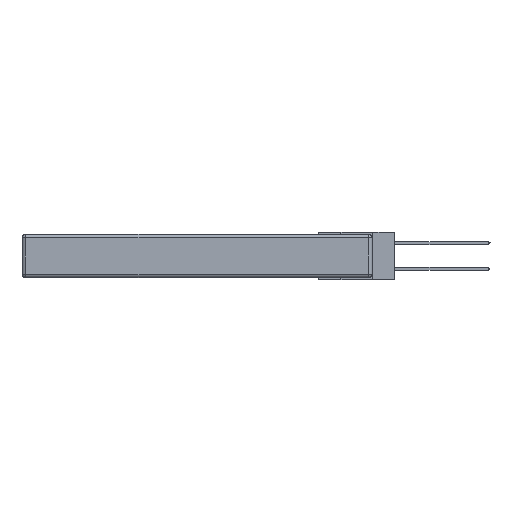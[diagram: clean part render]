
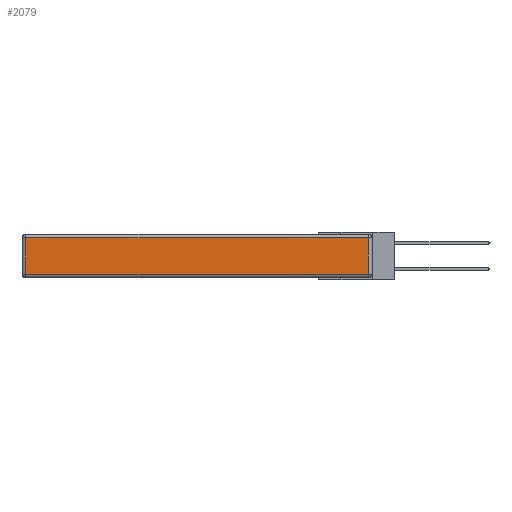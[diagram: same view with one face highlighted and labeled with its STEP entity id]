
A CAD part, left-side view. The second image highlights one B-rep face of the part: STEP entity #2079.
In plain terms, the highlighted planar face has unit normal (-1, 0, 0).
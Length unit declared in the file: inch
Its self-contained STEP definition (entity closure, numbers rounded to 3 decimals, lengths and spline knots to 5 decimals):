
#499 = DIRECTION ( 'NONE',  ( 0., 0., 1. ) ) ;
#761 = CARTESIAN_POINT ( 'NONE',  ( 0., 2.72, -0.313 ) ) ;
#2079 = ADVANCED_FACE ( 'NONE', ( #4059 ), #2693, .T. ) ;
#2693 = PLANE ( 'NONE',  #6199 ) ;
#4059 = FACE_OUTER_BOUND ( 'NONE', #22224, .T. ) ;
#5802 = DIRECTION ( 'NONE',  ( 0., 0., 1. ) ) ;
#6199 = AXIS2_PLACEMENT_3D ( 'NONE', #31024, #28366, #499 ) ;
#7087 = DIRECTION ( 'NONE',  ( 0., -1., 0. ) ) ;
#8063 = ORIENTED_EDGE ( 'NONE', *, *, #14645, .T. ) ;
#8081 = VECTOR ( 'NONE', #24309, 39.37008 ) ;
#8719 = CARTESIAN_POINT ( 'NONE',  ( 0., 0.03, -0.343 ) ) ;
#12425 = EDGE_CURVE ( 'NONE', #27812, #23654, #19739, .T. ) ;
#12857 = LINE ( 'NONE', #17059, #8081 ) ;
#12929 = LINE ( 'NONE', #8719, #15340 ) ;
#13012 = EDGE_CURVE ( 'NONE', #16909, #23980, #12929, .T. ) ;
#13393 = VECTOR ( 'NONE', #31324, 39.37008 ) ;
#14645 = EDGE_CURVE ( 'NONE', #23980, #27812, #12857, .T. ) ;
#15340 = VECTOR ( 'NONE', #5802, 39.37008 ) ;
#16909 = VERTEX_POINT ( 'NONE', #29527 ) ;
#17059 = CARTESIAN_POINT ( 'NONE',  ( 0., 2.75, -0.03 ) ) ;
#18660 = CARTESIAN_POINT ( 'NONE',  ( 0., 2.72, -0.343 ) ) ;
#19739 = LINE ( 'NONE', #18660, #13393 ) ;
#22224 = EDGE_LOOP ( 'NONE', ( #26022, #25964, #8063, #29429 ) ) ;
#22317 = CARTESIAN_POINT ( 'NONE',  ( 0., 0., -0.313 ) ) ;
#22921 = CARTESIAN_POINT ( 'NONE',  ( 0., 2.72, -0.03 ) ) ;
#23654 = VERTEX_POINT ( 'NONE', #761 ) ;
#23980 = VERTEX_POINT ( 'NONE', #29792 ) ;
#24309 = DIRECTION ( 'NONE',  ( 0., 1., 0. ) ) ;
#24898 = VECTOR ( 'NONE', #7087, 39.37008 ) ;
#25316 = LINE ( 'NONE', #22317, #24898 ) ;
#25964 = ORIENTED_EDGE ( 'NONE', *, *, #13012, .T. ) ;
#26022 = ORIENTED_EDGE ( 'NONE', *, *, #26476, .T. ) ;
#26476 = EDGE_CURVE ( 'NONE', #23654, #16909, #25316, .T. ) ;
#27812 = VERTEX_POINT ( 'NONE', #22921 ) ;
#28366 = DIRECTION ( 'NONE',  ( -1., 0., 0. ) ) ;
#29429 = ORIENTED_EDGE ( 'NONE', *, *, #12425, .T. ) ;
#29527 = CARTESIAN_POINT ( 'NONE',  ( 0., 0.03, -0.313 ) ) ;
#29792 = CARTESIAN_POINT ( 'NONE',  ( 0., 0.03, -0.03 ) ) ;
#31024 = CARTESIAN_POINT ( 'NONE',  ( 0., 0., -0.343 ) ) ;
#31324 = DIRECTION ( 'NONE',  ( 0., 0., -1. ) ) ;
